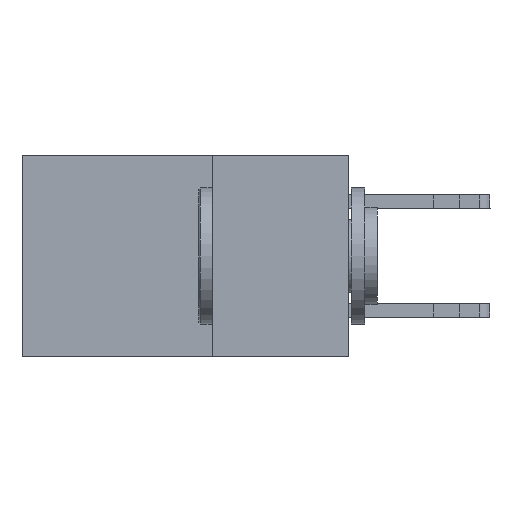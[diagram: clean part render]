
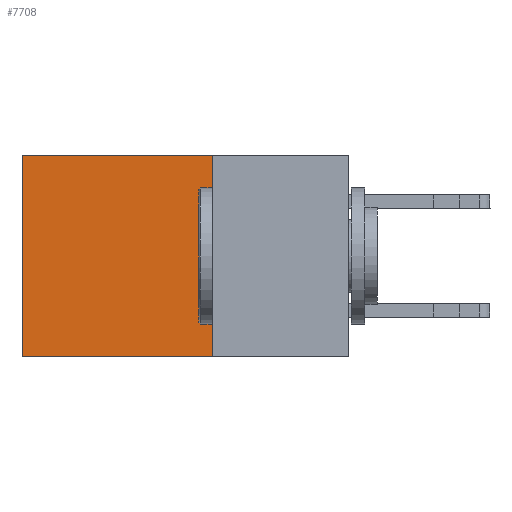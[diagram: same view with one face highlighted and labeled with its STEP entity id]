
A CAD part, left-side view. The second image highlights one B-rep face of the part: STEP entity #7708.
In plain terms, the highlighted planar face has unit normal (-1, 0, 0).
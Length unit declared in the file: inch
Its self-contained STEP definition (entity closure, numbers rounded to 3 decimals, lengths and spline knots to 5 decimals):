
#83 = EDGE_CURVE ( 'NONE', #3211, #3030, #4189, .T. ) ;
#546 = PLANE ( 'NONE',  #7097 ) ;
#1062 = VERTEX_POINT ( 'NONE', #3747 ) ;
#1121 = VECTOR ( 'NONE', #12773, 39.37008 ) ;
#3030 = VERTEX_POINT ( 'NONE', #11990 ) ;
#3146 = DIRECTION ( 'NONE',  ( 0., 1., 0. ) ) ;
#3211 = VERTEX_POINT ( 'NONE', #10580 ) ;
#3747 = CARTESIAN_POINT ( 'NONE',  ( 0.2615, 0.25, -0.37 ) ) ;
#3848 = FACE_OUTER_BOUND ( 'NONE', #12542, .T. ) ;
#4189 = LINE ( 'NONE', #13888, #1121 ) ;
#4623 = DIRECTION ( 'NONE',  ( 0., 0., -1. ) ) ;
#4921 = CARTESIAN_POINT ( 'NONE',  ( 0.2615, 0.25, -0.37 ) ) ;
#5156 = VERTEX_POINT ( 'NONE', #6664 ) ;
#6188 = ORIENTED_EDGE ( 'NONE', *, *, #14220, .F. ) ;
#6227 = LINE ( 'NONE', #6460, #12165 ) ;
#6344 = ORIENTED_EDGE ( 'NONE', *, *, #8510, .F. ) ;
#6460 = CARTESIAN_POINT ( 'NONE',  ( 0.2615, 0.25, -0.37 ) ) ;
#6664 = CARTESIAN_POINT ( 'NONE',  ( 0.2615, 0.6, -0.37 ) ) ;
#7010 = ORIENTED_EDGE ( 'NONE', *, *, #83, .T. ) ;
#7097 = AXIS2_PLACEMENT_3D ( 'NONE', #4921, #9360, #8284 ) ;
#7638 = DIRECTION ( 'NONE',  ( 0., 0., -1. ) ) ;
#7708 = ADVANCED_FACE ( 'NONE', ( #3848 ), #546, .F. ) ;
#7891 = CARTESIAN_POINT ( 'NONE',  ( 0.2615, 0.6, -0.37 ) ) ;
#8284 = DIRECTION ( 'NONE',  ( 0., 0., -1. ) ) ;
#8510 = EDGE_CURVE ( 'NONE', #3211, #1062, #6227, .T. ) ;
#9128 = VECTOR ( 'NONE', #4623, 39.37008 ) ;
#9147 = VECTOR ( 'NONE', #3146, 39.37008 ) ;
#9360 = DIRECTION ( 'NONE',  ( 1., 0., 0. ) ) ;
#10363 = ORIENTED_EDGE ( 'NONE', *, *, #13003, .T. ) ;
#10580 = CARTESIAN_POINT ( 'NONE',  ( 0.2615, 0.25, 0. ) ) ;
#11620 = CARTESIAN_POINT ( 'NONE',  ( 0.2615, 0.25, -0.37 ) ) ;
#11990 = CARTESIAN_POINT ( 'NONE',  ( 0.2615, 0.6, 0. ) ) ;
#12165 = VECTOR ( 'NONE', #7638, 39.37008 ) ;
#12542 = EDGE_LOOP ( 'NONE', ( #10363, #6188, #6344, #7010 ) ) ;
#12607 = LINE ( 'NONE', #11620, #9147 ) ;
#12773 = DIRECTION ( 'NONE',  ( 0., 1., 0. ) ) ;
#13003 = EDGE_CURVE ( 'NONE', #3030, #5156, #13504, .T. ) ;
#13504 = LINE ( 'NONE', #7891, #9128 ) ;
#13888 = CARTESIAN_POINT ( 'NONE',  ( 0.2615, 0.25, 0. ) ) ;
#14220 = EDGE_CURVE ( 'NONE', #1062, #5156, #12607, .T. ) ;
